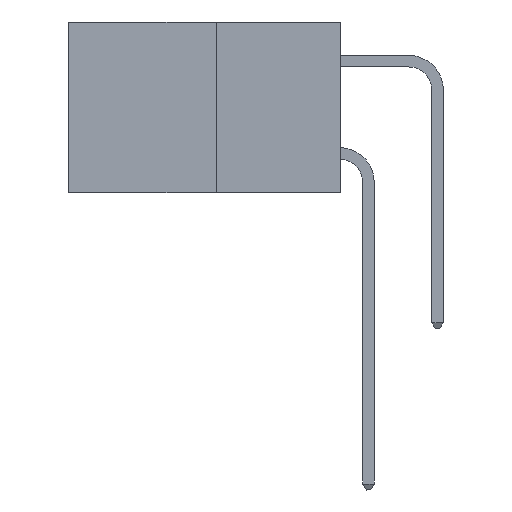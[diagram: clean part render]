
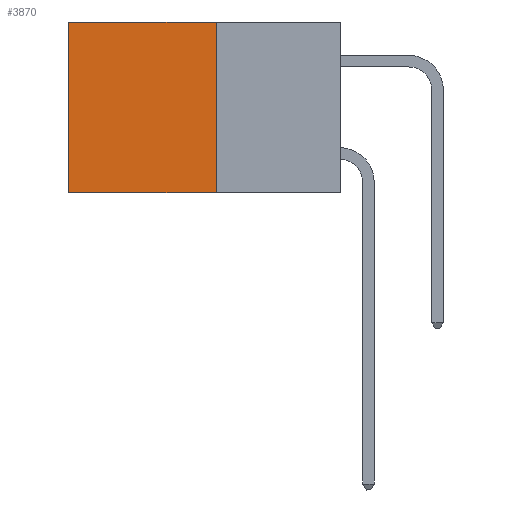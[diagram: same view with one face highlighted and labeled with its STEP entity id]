
A CAD part, left-side view. The second image highlights one B-rep face of the part: STEP entity #3870.
In plain terms, the highlighted planar face has unit normal (-1, 0, 0).
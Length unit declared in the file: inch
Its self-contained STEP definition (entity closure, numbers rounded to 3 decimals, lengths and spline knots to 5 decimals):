
#629 = AXIS2_PLACEMENT_3D ( 'NONE', #7607, #15117, #3885 ) ;
#2604 = ORIENTED_EDGE ( 'NONE', *, *, #13508, .F. ) ;
#3870 = ADVANCED_FACE ( 'NONE', ( #6162 ), #13239, .F. ) ;
#3885 = DIRECTION ( 'NONE',  ( 0., 0., -1. ) ) ;
#4632 = CARTESIAN_POINT ( 'NONE',  ( 0.277, 0.27, 0. ) ) ;
#4789 = DIRECTION ( 'NONE',  ( 0., 0., -1. ) ) ;
#4880 = VERTEX_POINT ( 'NONE', #17751 ) ;
#4927 = LINE ( 'NONE', #4632, #9933 ) ;
#6162 = FACE_OUTER_BOUND ( 'NONE', #20530, .T. ) ;
#6203 = CARTESIAN_POINT ( 'NONE',  ( 0.277, 0.27, -0.37 ) ) ;
#6534 = DIRECTION ( 'NONE',  ( 0., 1., 0. ) ) ;
#6695 = CARTESIAN_POINT ( 'NONE',  ( 0.277, 0.59, -0.37 ) ) ;
#7607 = CARTESIAN_POINT ( 'NONE',  ( 0.277, 0.27, -0.37 ) ) ;
#8476 = VECTOR ( 'NONE', #19726, 39.37008 ) ;
#8546 = CARTESIAN_POINT ( 'NONE',  ( 0.277, 0.27, -0.37 ) ) ;
#9446 = EDGE_CURVE ( 'NONE', #4880, #21968, #22573, .T. ) ;
#9933 = VECTOR ( 'NONE', #6534, 39.37008 ) ;
#10228 = CARTESIAN_POINT ( 'NONE',  ( 0.277, 0.27, -0.37 ) ) ;
#11164 = CARTESIAN_POINT ( 'NONE',  ( 0.277, 0.59, -0.37 ) ) ;
#11263 = CARTESIAN_POINT ( 'NONE',  ( 0.277, 0.27, 0. ) ) ;
#13239 = PLANE ( 'NONE',  #629 ) ;
#13441 = LINE ( 'NONE', #8546, #8476 ) ;
#13508 = EDGE_CURVE ( 'NONE', #24184, #23732, #17805, .T. ) ;
#13609 = EDGE_CURVE ( 'NONE', #24184, #4880, #4927, .T. ) ;
#13728 = DIRECTION ( 'NONE',  ( 0., 0., -1. ) ) ;
#13983 = ORIENTED_EDGE ( 'NONE', *, *, #9446, .T. ) ;
#15117 = DIRECTION ( 'NONE',  ( 1., 0., 0. ) ) ;
#17751 = CARTESIAN_POINT ( 'NONE',  ( 0.277, 0.59, 0. ) ) ;
#17805 = LINE ( 'NONE', #6203, #21605 ) ;
#18651 = ORIENTED_EDGE ( 'NONE', *, *, #13609, .T. ) ;
#19704 = EDGE_CURVE ( 'NONE', #23732, #21968, #13441, .T. ) ;
#19726 = DIRECTION ( 'NONE',  ( 0., 1., 0. ) ) ;
#20271 = ORIENTED_EDGE ( 'NONE', *, *, #19704, .F. ) ;
#20530 = EDGE_LOOP ( 'NONE', ( #13983, #20271, #2604, #18651 ) ) ;
#21605 = VECTOR ( 'NONE', #13728, 39.37008 ) ;
#21968 = VERTEX_POINT ( 'NONE', #11164 ) ;
#22000 = VECTOR ( 'NONE', #4789, 39.37008 ) ;
#22573 = LINE ( 'NONE', #6695, #22000 ) ;
#23732 = VERTEX_POINT ( 'NONE', #10228 ) ;
#24184 = VERTEX_POINT ( 'NONE', #11263 ) ;
